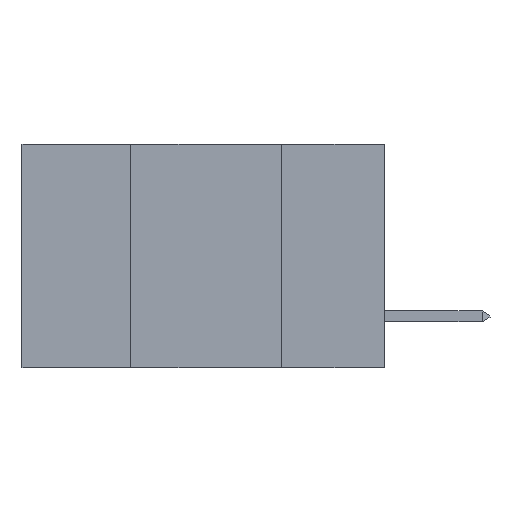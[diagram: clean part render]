
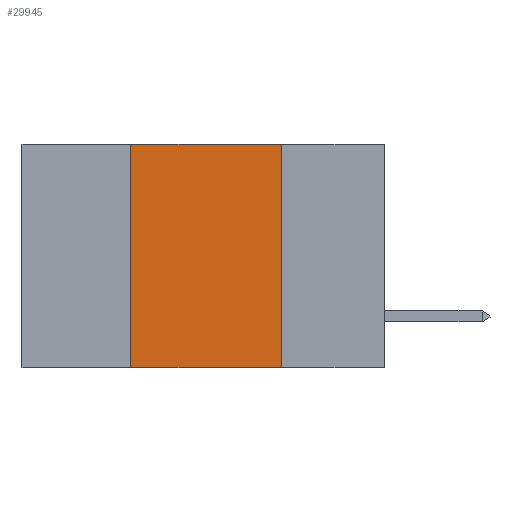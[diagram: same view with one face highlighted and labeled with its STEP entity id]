
A CAD part, left-side view. The second image highlights one B-rep face of the part: STEP entity #29945.
In plain terms, the highlighted planar face has unit normal (-1, 0, 0).
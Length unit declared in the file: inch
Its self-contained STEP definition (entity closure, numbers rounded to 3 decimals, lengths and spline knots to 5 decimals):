
#144 = CARTESIAN_POINT ( 'NONE',  ( 0., 0.6, 0. ) ) ;
#944 = ORIENTED_EDGE ( 'NONE', *, *, #26373, .F. ) ;
#1584 = CARTESIAN_POINT ( 'NONE',  ( 0., 0.17, 0. ) ) ;
#2466 = VERTEX_POINT ( 'NONE', #6477 ) ;
#4298 = ORIENTED_EDGE ( 'NONE', *, *, #14791, .T. ) ;
#6477 = CARTESIAN_POINT ( 'NONE',  ( 0., 0.42, 0. ) ) ;
#6763 = VECTOR ( 'NONE', #32930, 39.37008 ) ;
#7560 = ORIENTED_EDGE ( 'NONE', *, *, #22296, .F. ) ;
#7604 = PLANE ( 'NONE',  #23440 ) ;
#8134 = DIRECTION ( 'NONE',  ( 0., -1., 0. ) ) ;
#8372 = VECTOR ( 'NONE', #17537, 39.37008 ) ;
#10108 = ORIENTED_EDGE ( 'NONE', *, *, #17674, .F. ) ;
#10306 = CARTESIAN_POINT ( 'NONE',  ( 0., 0.6, 0. ) ) ;
#10482 = EDGE_LOOP ( 'NONE', ( #7560, #944, #10108, #4298 ) ) ;
#10594 = VERTEX_POINT ( 'NONE', #1584 ) ;
#12975 = DIRECTION ( 'NONE',  ( 0., 0., -1. ) ) ;
#14348 = CARTESIAN_POINT ( 'NONE',  ( 0., 0.17, 0. ) ) ;
#14662 = LINE ( 'NONE', #14348, #6763 ) ;
#14791 = EDGE_CURVE ( 'NONE', #18643, #29193, #34275, .T. ) ;
#17537 = DIRECTION ( 'NONE',  ( 0., 0., 1. ) ) ;
#17674 = EDGE_CURVE ( 'NONE', #18643, #2466, #29538, .T. ) ;
#18415 = VECTOR ( 'NONE', #8134, 39.37008 ) ;
#18643 = VERTEX_POINT ( 'NONE', #18987 ) ;
#18987 = CARTESIAN_POINT ( 'NONE',  ( 0., 0.42, -0.37 ) ) ;
#22296 = EDGE_CURVE ( 'NONE', #10594, #29193, #14662, .T. ) ;
#22300 = FACE_OUTER_BOUND ( 'NONE', #10482, .T. ) ;
#23440 = AXIS2_PLACEMENT_3D ( 'NONE', #10306, #28818, #12975 ) ;
#25577 = VECTOR ( 'NONE', #33657, 39.37008 ) ;
#25689 = CARTESIAN_POINT ( 'NONE',  ( 0., 0.6, -0.37 ) ) ;
#26373 = EDGE_CURVE ( 'NONE', #2466, #10594, #32463, .T. ) ;
#28818 = DIRECTION ( 'NONE',  ( 1., 0., 0. ) ) ;
#29193 = VERTEX_POINT ( 'NONE', #33573 ) ;
#29538 = LINE ( 'NONE', #30723, #8372 ) ;
#29945 = ADVANCED_FACE ( 'NONE', ( #22300 ), #7604, .F. ) ;
#30723 = CARTESIAN_POINT ( 'NONE',  ( 0., 0.42, 0. ) ) ;
#32463 = LINE ( 'NONE', #144, #18415 ) ;
#32930 = DIRECTION ( 'NONE',  ( 0., 0., -1. ) ) ;
#33573 = CARTESIAN_POINT ( 'NONE',  ( 0., 0.17, -0.37 ) ) ;
#33657 = DIRECTION ( 'NONE',  ( 0., -1., 0. ) ) ;
#34275 = LINE ( 'NONE', #25689, #25577 ) ;
